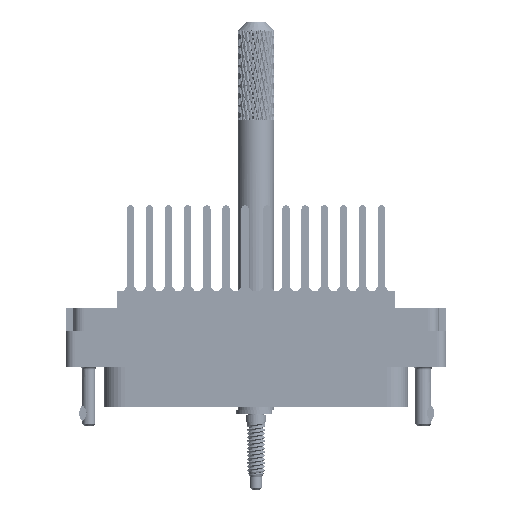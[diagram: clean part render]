
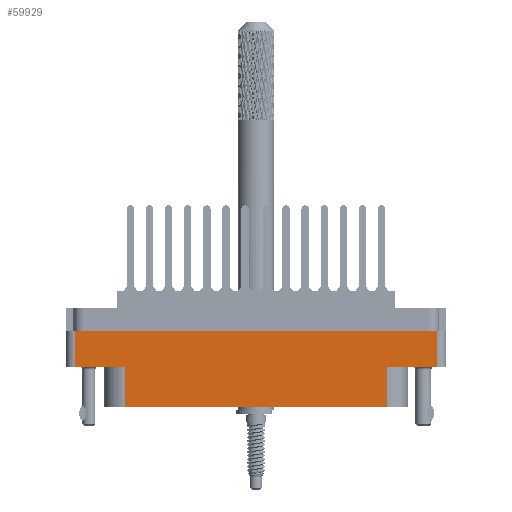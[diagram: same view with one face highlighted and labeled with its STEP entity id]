
A CAD part, front view. The second image highlights one B-rep face of the part: STEP entity #59929.
In plain terms, the highlighted planar face has unit normal (0, -1, 0).
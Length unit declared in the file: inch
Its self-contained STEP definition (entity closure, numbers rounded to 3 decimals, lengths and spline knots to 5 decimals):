
#4232 = CARTESIAN_POINT ( 'NONE',  ( -0.895, -0.438, -0.789 ) ) ;
#4814 = DIRECTION ( 'NONE',  ( 0., 0., -1. ) ) ;
#5111 = DIRECTION ( 'NONE',  ( 0., -1., 0. ) ) ;
#5683 = EDGE_CURVE ( 'NONE', #21754, #81600, #24499, .T. ) ;
#10648 = CARTESIAN_POINT ( 'NONE',  ( -0.895, -0.438, -0.52 ) ) ;
#10688 = LINE ( 'NONE', #60888, #95032 ) ;
#11286 = CARTESIAN_POINT ( 'NONE',  ( -0.895, -0.438, -0.789 ) ) ;
#11673 = DIRECTION ( 'NONE',  ( 1., 0., 0. ) ) ;
#16305 = CARTESIAN_POINT ( 'NONE',  ( -1.2335, -0.438, -0.52 ) ) ;
#16844 = VECTOR ( 'NONE', #4814, 39.37008 ) ;
#16983 = CARTESIAN_POINT ( 'NONE',  ( 0.895, -0.438, -0.52 ) ) ;
#17357 = ORIENTED_EDGE ( 'NONE', *, *, #120625, .F. ) ;
#18091 = VECTOR ( 'NONE', #55775, 39.37008 ) ;
#18627 = EDGE_LOOP ( 'NONE', ( #78394, #64013, #82620, #105879, #68887, #83735, #17357, #73411 ) ) ;
#21754 = VERTEX_POINT ( 'NONE', #10648 ) ;
#24499 = LINE ( 'NONE', #4232, #117692 ) ;
#27376 = LINE ( 'NONE', #62023, #16844 ) ;
#35958 = VERTEX_POINT ( 'NONE', #47428 ) ;
#35960 = DIRECTION ( 'NONE',  ( 0., 0., 1. ) ) ;
#46669 = VERTEX_POINT ( 'NONE', #16305 ) ;
#47402 = CARTESIAN_POINT ( 'NONE',  ( 1.2335, -0.438, -0.52 ) ) ;
#47428 = CARTESIAN_POINT ( 'NONE',  ( 0.895, -0.438, -0.789 ) ) ;
#51784 = VECTOR ( 'NONE', #79375, 39.37008 ) ;
#52594 = EDGE_CURVE ( 'NONE', #81600, #35958, #94652, .T. ) ;
#55309 = CARTESIAN_POINT ( 'NONE',  ( -1.2955, -0.438, -0.789 ) ) ;
#55775 = DIRECTION ( 'NONE',  ( -1., 0., 0. ) ) ;
#56578 = VERTEX_POINT ( 'NONE', #103672 ) ;
#57124 = EDGE_CURVE ( 'NONE', #75563, #111147, #111954, .T. ) ;
#59929 = ADVANCED_FACE ( 'NONE', ( #104058 ), #119034, .T. ) ;
#60888 = CARTESIAN_POINT ( 'NONE',  ( 0., -0.438, -0.274 ) ) ;
#61629 = CARTESIAN_POINT ( 'NONE',  ( 1.2335, -0.438, -0.789 ) ) ;
#62023 = CARTESIAN_POINT ( 'NONE',  ( -1.2335, -0.438, -0.789 ) ) ;
#62718 = CARTESIAN_POINT ( 'NONE',  ( -1.2955, -0.438, -0.789 ) ) ;
#64013 = ORIENTED_EDGE ( 'NONE', *, *, #89228, .T. ) ;
#64989 = AXIS2_PLACEMENT_3D ( 'NONE', #62718, #5111, #90945 ) ;
#65686 = CARTESIAN_POINT ( 'NONE',  ( -1.2335, -0.438, -0.274 ) ) ;
#68515 = CARTESIAN_POINT ( 'NONE',  ( 0., -0.438, -0.52 ) ) ;
#68887 = ORIENTED_EDGE ( 'NONE', *, *, #52594, .T. ) ;
#71605 = VERTEX_POINT ( 'NONE', #65686 ) ;
#72332 = DIRECTION ( 'NONE',  ( 0., 0., -1. ) ) ;
#72404 = EDGE_CURVE ( 'NONE', #35958, #56578, #102205, .T. ) ;
#73411 = ORIENTED_EDGE ( 'NONE', *, *, #57124, .T. ) ;
#74741 = CARTESIAN_POINT ( 'NONE',  ( 1.2335, -0.438, -0.274 ) ) ;
#75301 = LINE ( 'NONE', #114207, #18091 ) ;
#75563 = VERTEX_POINT ( 'NONE', #47402 ) ;
#78394 = ORIENTED_EDGE ( 'NONE', *, *, #110887, .F. ) ;
#79375 = DIRECTION ( 'NONE',  ( 0., 0., 1. ) ) ;
#81600 = VERTEX_POINT ( 'NONE', #11286 ) ;
#82620 = ORIENTED_EDGE ( 'NONE', *, *, #121730, .F. ) ;
#83735 = ORIENTED_EDGE ( 'NONE', *, *, #72404, .T. ) ;
#87877 = DIRECTION ( 'NONE',  ( -1., 0., 0. ) ) ;
#89228 = EDGE_CURVE ( 'NONE', #71605, #46669, #27376, .T. ) ;
#90511 = LINE ( 'NONE', #68515, #117453 ) ;
#90945 = DIRECTION ( 'NONE',  ( 0., 0., -1. ) ) ;
#94652 = LINE ( 'NONE', #55309, #111085 ) ;
#95032 = VECTOR ( 'NONE', #11673, 39.37008 ) ;
#102205 = LINE ( 'NONE', #16983, #115663 ) ;
#103672 = CARTESIAN_POINT ( 'NONE',  ( 0.895, -0.438, -0.52 ) ) ;
#104058 = FACE_OUTER_BOUND ( 'NONE', #18627, .T. ) ;
#105879 = ORIENTED_EDGE ( 'NONE', *, *, #5683, .T. ) ;
#110887 = EDGE_CURVE ( 'NONE', #71605, #111147, #10688, .T. ) ;
#111085 = VECTOR ( 'NONE', #122913, 39.37008 ) ;
#111147 = VERTEX_POINT ( 'NONE', #74741 ) ;
#111954 = LINE ( 'NONE', #61629, #51784 ) ;
#114207 = CARTESIAN_POINT ( 'NONE',  ( 0., -0.438, -0.52 ) ) ;
#115663 = VECTOR ( 'NONE', #35960, 39.37008 ) ;
#117453 = VECTOR ( 'NONE', #87877, 39.37008 ) ;
#117692 = VECTOR ( 'NONE', #72332, 39.37008 ) ;
#119034 = PLANE ( 'NONE',  #64989 ) ;
#120625 = EDGE_CURVE ( 'NONE', #75563, #56578, #90511, .T. ) ;
#121730 = EDGE_CURVE ( 'NONE', #21754, #46669, #75301, .T. ) ;
#122913 = DIRECTION ( 'NONE',  ( 1., 0., 0. ) ) ;
